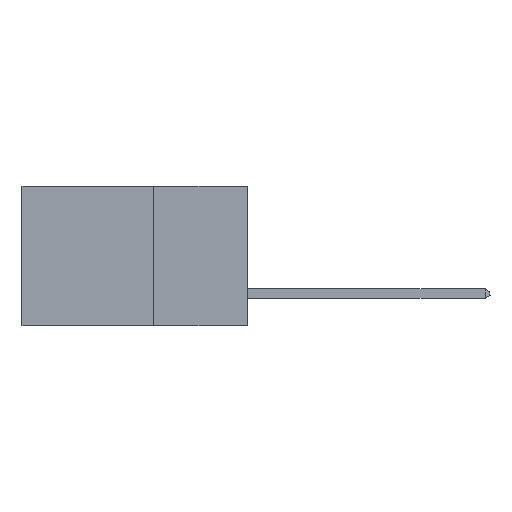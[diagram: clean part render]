
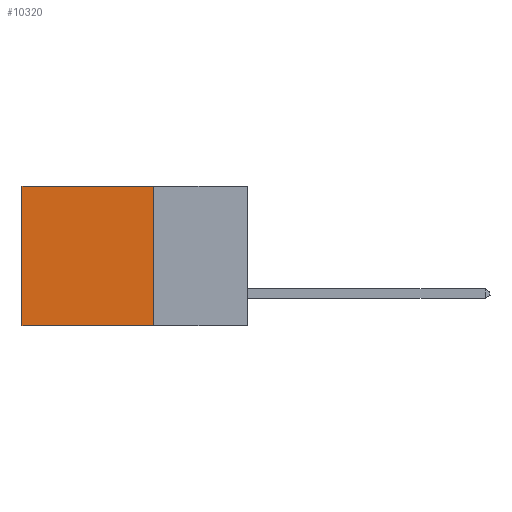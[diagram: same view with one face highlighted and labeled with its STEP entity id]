
A CAD part, left-side view. The second image highlights one B-rep face of the part: STEP entity #10320.
In plain terms, the highlighted planar face has unit normal (-1, 0, 0).
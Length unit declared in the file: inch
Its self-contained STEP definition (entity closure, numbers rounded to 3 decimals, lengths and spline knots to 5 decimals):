
#161 = ORIENTED_EDGE ( 'NONE', *, *, #355, .F. ) ;
#355 = EDGE_CURVE ( 'NONE', #8300, #22239, #3509, .T. ) ;
#3509 = LINE ( 'NONE', #17188, #15385 ) ;
#4283 = CARTESIAN_POINT ( 'NONE',  ( 0.298, 0.25, -0.37 ) ) ;
#5509 = VERTEX_POINT ( 'NONE', #29794 ) ;
#6710 = DIRECTION ( 'NONE',  ( 0., 1., 0. ) ) ;
#7145 = DIRECTION ( 'NONE',  ( 1., 0., 0. ) ) ;
#8300 = VERTEX_POINT ( 'NONE', #28958 ) ;
#9033 = ORIENTED_EDGE ( 'NONE', *, *, #23795, .T. ) ;
#9137 = CARTESIAN_POINT ( 'NONE',  ( 0.298, 0.25, -0.37 ) ) ;
#9443 = VECTOR ( 'NONE', #10579, 39.37008 ) ;
#10320 = ADVANCED_FACE ( 'NONE', ( #28292 ), #21199, .F. ) ;
#10579 = DIRECTION ( 'NONE',  ( 0., 0., -1. ) ) ;
#11015 = VECTOR ( 'NONE', #28700, 39.37008 ) ;
#11093 = EDGE_CURVE ( 'NONE', #8300, #25732, #17238, .T. ) ;
#14183 = EDGE_CURVE ( 'NONE', #22239, #5509, #16255, .T. ) ;
#14334 = ORIENTED_EDGE ( 'NONE', *, *, #11093, .T. ) ;
#14805 = VECTOR ( 'NONE', #6710, 39.37008 ) ;
#14815 = AXIS2_PLACEMENT_3D ( 'NONE', #28135, #7145, #23538 ) ;
#15385 = VECTOR ( 'NONE', #18150, 39.37008 ) ;
#15654 = LINE ( 'NONE', #19873, #9443 ) ;
#16255 = LINE ( 'NONE', #4283, #14805 ) ;
#17188 = CARTESIAN_POINT ( 'NONE',  ( 0.298, 0.25, 0. ) ) ;
#17238 = LINE ( 'NONE', #26348, #11015 ) ;
#18150 = DIRECTION ( 'NONE',  ( 0., 0., -1. ) ) ;
#19873 = CARTESIAN_POINT ( 'NONE',  ( 0.298, 0.6, 0. ) ) ;
#20313 = CARTESIAN_POINT ( 'NONE',  ( 0.298, 0.6, 0. ) ) ;
#21199 = PLANE ( 'NONE',  #14815 ) ;
#22239 = VERTEX_POINT ( 'NONE', #9137 ) ;
#23538 = DIRECTION ( 'NONE',  ( 0., 0., -1. ) ) ;
#23795 = EDGE_CURVE ( 'NONE', #25732, #5509, #15654, .T. ) ;
#25732 = VERTEX_POINT ( 'NONE', #20313 ) ;
#26048 = EDGE_LOOP ( 'NONE', ( #9033, #26538, #161, #14334 ) ) ;
#26348 = CARTESIAN_POINT ( 'NONE',  ( 0.298, 0.25, 0. ) ) ;
#26538 = ORIENTED_EDGE ( 'NONE', *, *, #14183, .F. ) ;
#28135 = CARTESIAN_POINT ( 'NONE',  ( 0.298, 0.25, 0. ) ) ;
#28292 = FACE_OUTER_BOUND ( 'NONE', #26048, .T. ) ;
#28700 = DIRECTION ( 'NONE',  ( 0., 1., 0. ) ) ;
#28958 = CARTESIAN_POINT ( 'NONE',  ( 0.298, 0.25, 0. ) ) ;
#29794 = CARTESIAN_POINT ( 'NONE',  ( 0.298, 0.6, -0.37 ) ) ;
